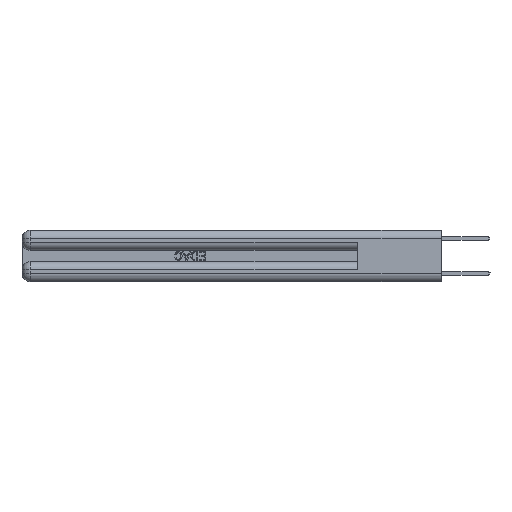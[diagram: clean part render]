
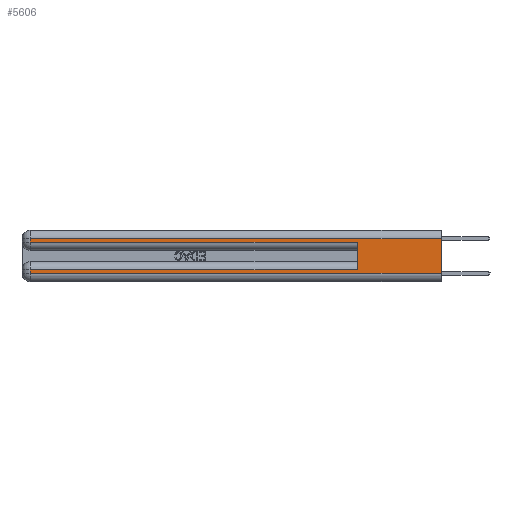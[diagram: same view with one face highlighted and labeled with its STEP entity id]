
A CAD part, left-side view. The second image highlights one B-rep face of the part: STEP entity #5606.
In plain terms, the highlighted planar face has unit normal (-1, 0, 0).
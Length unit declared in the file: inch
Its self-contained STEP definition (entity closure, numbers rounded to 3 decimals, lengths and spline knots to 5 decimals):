
#87 = CARTESIAN_POINT ( 'NONE',  ( 0., 0., 0.31 ) ) ;
#126 = VERTEX_POINT ( 'NONE', #10435 ) ;
#392 = DIRECTION ( 'NONE',  ( 0., 1., 0. ) ) ;
#548 = EDGE_CURVE ( 'NONE', #7947, #15564, #18539, .T. ) ;
#1201 = VECTOR ( 'NONE', #12673, 39.37008 ) ;
#1890 = LINE ( 'NONE', #27189, #1201 ) ;
#2449 = CARTESIAN_POINT ( 'NONE',  ( 0., 2.94, 0.37 ) ) ;
#2528 = LINE ( 'NONE', #26388, #6680 ) ;
#2530 = ORIENTED_EDGE ( 'NONE', *, *, #7248, .T. ) ;
#2726 = DIRECTION ( 'NONE',  ( 1., 0., 0. ) ) ;
#2836 = VECTOR ( 'NONE', #4588, 39.37008 ) ;
#2922 = VERTEX_POINT ( 'NONE', #24291 ) ;
#3355 = LINE ( 'NONE', #15289, #4057 ) ;
#4057 = VECTOR ( 'NONE', #22554, 39.37008 ) ;
#4588 = DIRECTION ( 'NONE',  ( 0., 0., -1. ) ) ;
#4828 = CARTESIAN_POINT ( 'NONE',  ( 0., 2.94, 0.285 ) ) ;
#5606 = ADVANCED_FACE ( 'NONE', ( #14452 ), #26824, .F. ) ;
#5955 = VERTEX_POINT ( 'NONE', #6068 ) ;
#6068 = CARTESIAN_POINT ( 'NONE',  ( 0., 0.6, 0.285 ) ) ;
#6351 = CARTESIAN_POINT ( 'NONE',  ( 0., 2.94, 0.085 ) ) ;
#6571 = VERTEX_POINT ( 'NONE', #9227 ) ;
#6680 = VECTOR ( 'NONE', #15360, 39.37008 ) ;
#7236 = EDGE_CURVE ( 'NONE', #126, #8096, #16074, .T. ) ;
#7248 = EDGE_CURVE ( 'NONE', #18982, #5955, #3355, .T. ) ;
#7947 = VERTEX_POINT ( 'NONE', #20753 ) ;
#8096 = VERTEX_POINT ( 'NONE', #14448 ) ;
#8845 = ORIENTED_EDGE ( 'NONE', *, *, #13608, .F. ) ;
#9120 = ORIENTED_EDGE ( 'NONE', *, *, #7236, .T. ) ;
#9227 = CARTESIAN_POINT ( 'NONE',  ( 0., 2.94, 0.06 ) ) ;
#10435 = CARTESIAN_POINT ( 'NONE',  ( 0., 0., 0.31 ) ) ;
#12614 = LINE ( 'NONE', #18911, #22550 ) ;
#12673 = DIRECTION ( 'NONE',  ( 0., -1., 0. ) ) ;
#13608 = EDGE_CURVE ( 'NONE', #7947, #5955, #2528, .T. ) ;
#13663 = DIRECTION ( 'NONE',  ( 0., 0., -1. ) ) ;
#13779 = VECTOR ( 'NONE', #13663, 39.37008 ) ;
#13872 = CARTESIAN_POINT ( 'NONE',  ( 0., 0., 0.37 ) ) ;
#14448 = CARTESIAN_POINT ( 'NONE',  ( 0., 2.94, 0.31 ) ) ;
#14452 = FACE_OUTER_BOUND ( 'NONE', #28277, .T. ) ;
#15194 = DIRECTION ( 'NONE',  ( 0., 1., 0. ) ) ;
#15289 = CARTESIAN_POINT ( 'NONE',  ( 0., 0., 0.285 ) ) ;
#15360 = DIRECTION ( 'NONE',  ( 0., 0., 1. ) ) ;
#15564 = VERTEX_POINT ( 'NONE', #6351 ) ;
#16074 = LINE ( 'NONE', #87, #17793 ) ;
#16907 = ORIENTED_EDGE ( 'NONE', *, *, #21411, .T. ) ;
#17183 = VECTOR ( 'NONE', #15194, 39.37008 ) ;
#17793 = VECTOR ( 'NONE', #392, 39.37008 ) ;
#18539 = LINE ( 'NONE', #28377, #17183 ) ;
#18911 = CARTESIAN_POINT ( 'NONE',  ( 0., 2.94, 0.37 ) ) ;
#18982 = VERTEX_POINT ( 'NONE', #4828 ) ;
#19235 = EDGE_CURVE ( 'NONE', #126, #2922, #25419, .T. ) ;
#20753 = CARTESIAN_POINT ( 'NONE',  ( 0., 0.6, 0.085 ) ) ;
#21411 = EDGE_CURVE ( 'NONE', #15564, #6571, #12614, .T. ) ;
#21578 = ORIENTED_EDGE ( 'NONE', *, *, #22017, .T. ) ;
#22017 = EDGE_CURVE ( 'NONE', #6571, #2922, #1890, .T. ) ;
#22350 = CARTESIAN_POINT ( 'NONE',  ( 0., 0., 0.37 ) ) ;
#22550 = VECTOR ( 'NONE', #28110, 39.37008 ) ;
#22554 = DIRECTION ( 'NONE',  ( 0., -1., 0. ) ) ;
#22660 = DIRECTION ( 'NONE',  ( 0., 0., -1. ) ) ;
#22898 = AXIS2_PLACEMENT_3D ( 'NONE', #13872, #2726, #22660 ) ;
#23095 = LINE ( 'NONE', #2449, #2836 ) ;
#23285 = EDGE_CURVE ( 'NONE', #8096, #18982, #23095, .T. ) ;
#24291 = CARTESIAN_POINT ( 'NONE',  ( 0., 0., 0.06 ) ) ;
#24686 = ORIENTED_EDGE ( 'NONE', *, *, #548, .T. ) ;
#25419 = LINE ( 'NONE', #22350, #13779 ) ;
#26388 = CARTESIAN_POINT ( 'NONE',  ( 0., 0.6, 0.145 ) ) ;
#26559 = ORIENTED_EDGE ( 'NONE', *, *, #23285, .T. ) ;
#26824 = PLANE ( 'NONE',  #22898 ) ;
#27189 = CARTESIAN_POINT ( 'NONE',  ( 0., 0., 0.06 ) ) ;
#28022 = ORIENTED_EDGE ( 'NONE', *, *, #19235, .F. ) ;
#28110 = DIRECTION ( 'NONE',  ( 0., 0., -1. ) ) ;
#28277 = EDGE_LOOP ( 'NONE', ( #28022, #9120, #26559, #2530, #8845, #24686, #16907, #21578 ) ) ;
#28377 = CARTESIAN_POINT ( 'NONE',  ( 0., 0., 0.085 ) ) ;
